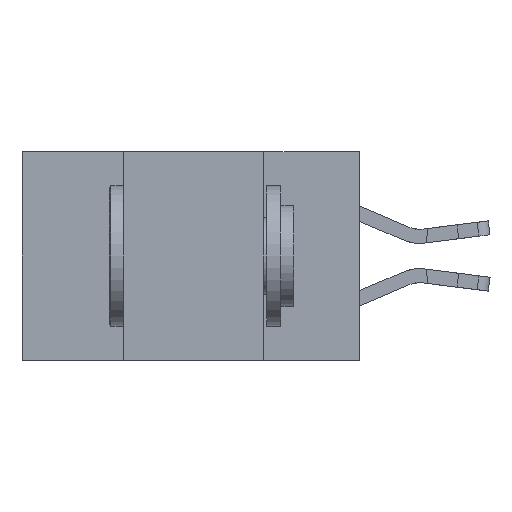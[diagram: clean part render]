
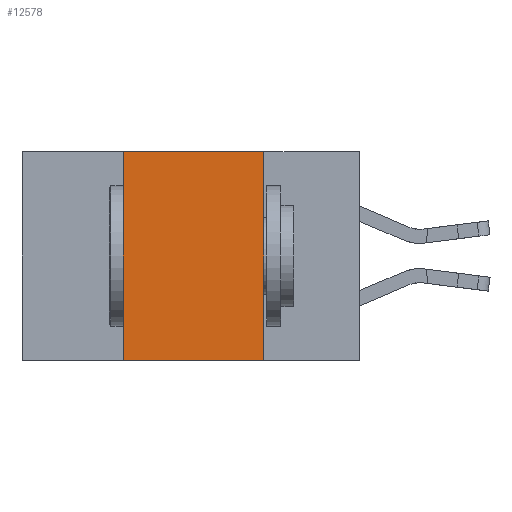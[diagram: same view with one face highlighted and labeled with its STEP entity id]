
A CAD part, left-side view. The second image highlights one B-rep face of the part: STEP entity #12578.
In plain terms, the highlighted planar face has unit normal (-1, 0, 0).
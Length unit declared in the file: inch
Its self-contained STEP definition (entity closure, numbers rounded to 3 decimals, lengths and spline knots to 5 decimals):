
#118 = CARTESIAN_POINT ( 'NONE',  ( 0., 0.6, 0. ) ) ;
#325 = DIRECTION ( 'NONE',  ( 0., -1., 0. ) ) ;
#1217 = VERTEX_POINT ( 'NONE', #21674 ) ;
#1931 = DIRECTION ( 'NONE',  ( 0., 0., -1. ) ) ;
#3164 = DIRECTION ( 'NONE',  ( 0., 0., -1. ) ) ;
#6477 = EDGE_CURVE ( 'NONE', #19095, #19074, #16046, .T. ) ;
#6707 = CARTESIAN_POINT ( 'NONE',  ( 0., 0.42, 0. ) ) ;
#6824 = CARTESIAN_POINT ( 'NONE',  ( 0., 0.17, 0. ) ) ;
#7260 = ORIENTED_EDGE ( 'NONE', *, *, #17673, .T. ) ;
#7696 = VECTOR ( 'NONE', #3164, 39.37008 ) ;
#7782 = VECTOR ( 'NONE', #11617, 39.37008 ) ;
#7898 = CARTESIAN_POINT ( 'NONE',  ( 0., 0.17, 0. ) ) ;
#8440 = EDGE_CURVE ( 'NONE', #1217, #20821, #19906, .T. ) ;
#9068 = DIRECTION ( 'NONE',  ( 1., 0., 0. ) ) ;
#11617 = DIRECTION ( 'NONE',  ( 0., 0., 1. ) ) ;
#11978 = FACE_OUTER_BOUND ( 'NONE', #17114, .T. ) ;
#12028 = CARTESIAN_POINT ( 'NONE',  ( 0., 0.17, -0.37 ) ) ;
#12578 = ADVANCED_FACE ( 'NONE', ( #11978 ), #17626, .F. ) ;
#13542 = ORIENTED_EDGE ( 'NONE', *, *, #21739, .F. ) ;
#14195 = VECTOR ( 'NONE', #325, 39.37008 ) ;
#15190 = AXIS2_PLACEMENT_3D ( 'NONE', #17553, #9068, #1931 ) ;
#15316 = ORIENTED_EDGE ( 'NONE', *, *, #8440, .F. ) ;
#15572 = CARTESIAN_POINT ( 'NONE',  ( 0., 0.42, 0. ) ) ;
#16046 = LINE ( 'NONE', #7898, #7696 ) ;
#17114 = EDGE_LOOP ( 'NONE', ( #20575, #13542, #15316, #7260 ) ) ;
#17553 = CARTESIAN_POINT ( 'NONE',  ( 0., 0.6, 0. ) ) ;
#17610 = VECTOR ( 'NONE', #20307, 39.37008 ) ;
#17626 = PLANE ( 'NONE',  #15190 ) ;
#17673 = EDGE_CURVE ( 'NONE', #1217, #19074, #19755, .T. ) ;
#18589 = CARTESIAN_POINT ( 'NONE',  ( 0., 0.6, -0.37 ) ) ;
#18778 = LINE ( 'NONE', #118, #14195 ) ;
#19074 = VERTEX_POINT ( 'NONE', #12028 ) ;
#19095 = VERTEX_POINT ( 'NONE', #6824 ) ;
#19755 = LINE ( 'NONE', #18589, #17610 ) ;
#19906 = LINE ( 'NONE', #6707, #7782 ) ;
#20307 = DIRECTION ( 'NONE',  ( 0., -1., 0. ) ) ;
#20575 = ORIENTED_EDGE ( 'NONE', *, *, #6477, .F. ) ;
#20821 = VERTEX_POINT ( 'NONE', #15572 ) ;
#21674 = CARTESIAN_POINT ( 'NONE',  ( 0., 0.42, -0.37 ) ) ;
#21739 = EDGE_CURVE ( 'NONE', #20821, #19095, #18778, .T. ) ;
